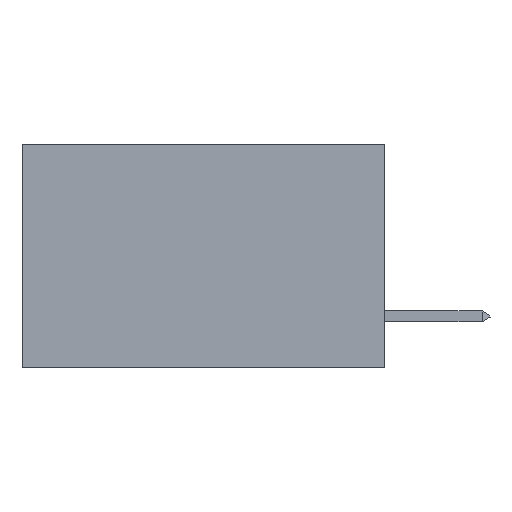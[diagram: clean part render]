
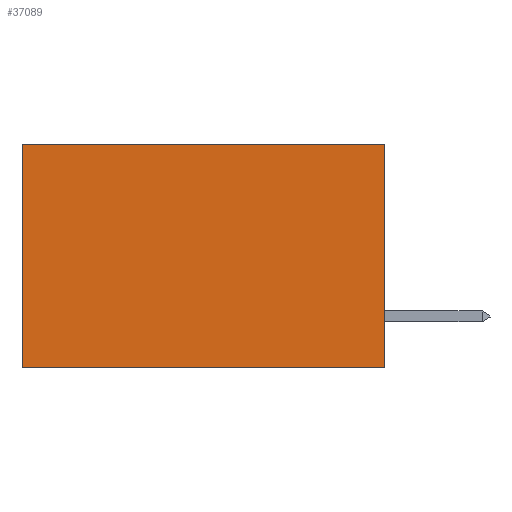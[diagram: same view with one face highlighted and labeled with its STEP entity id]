
A CAD part, left-side view. The second image highlights one B-rep face of the part: STEP entity #37089.
In plain terms, the highlighted planar face has unit normal (-1, 0, 0).
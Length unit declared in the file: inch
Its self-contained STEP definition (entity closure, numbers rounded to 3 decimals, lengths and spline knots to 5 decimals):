
#226 = VERTEX_POINT ( 'NONE', #22843 ) ;
#291 = EDGE_CURVE ( 'NONE', #226, #2371, #13985, .T. ) ;
#1689 = EDGE_CURVE ( 'NONE', #10957, #2266, #26819, .T. ) ;
#2266 = VERTEX_POINT ( 'NONE', #9314 ) ;
#2371 = VERTEX_POINT ( 'NONE', #36547 ) ;
#2788 = ORIENTED_EDGE ( 'NONE', *, *, #1689, .F. ) ;
#2862 = DIRECTION ( 'NONE',  ( 0., 1., 0. ) ) ;
#5697 = LINE ( 'NONE', #27568, #25083 ) ;
#6122 = VECTOR ( 'NONE', #29464, 39.37008 ) ;
#6258 = EDGE_CURVE ( 'NONE', #226, #10957, #12650, .T. ) ;
#7925 = VECTOR ( 'NONE', #2862, 39.37008 ) ;
#8088 = CARTESIAN_POINT ( 'NONE',  ( 0.2875, 0., 0. ) ) ;
#9281 = CARTESIAN_POINT ( 'NONE',  ( 0.2875, 0., 0. ) ) ;
#9314 = CARTESIAN_POINT ( 'NONE',  ( 0.2875, 0.6, -0.37 ) ) ;
#9414 = DIRECTION ( 'NONE',  ( 1., 0., 0. ) ) ;
#9442 = VECTOR ( 'NONE', #23203, 39.37008 ) ;
#10364 = EDGE_CURVE ( 'NONE', #2371, #2266, #5697, .T. ) ;
#10585 = AXIS2_PLACEMENT_3D ( 'NONE', #9281, #9414, #29899 ) ;
#10957 = VERTEX_POINT ( 'NONE', #12970 ) ;
#12650 = LINE ( 'NONE', #8088, #9442 ) ;
#12970 = CARTESIAN_POINT ( 'NONE',  ( 0.2875, 0., -0.37 ) ) ;
#13985 = LINE ( 'NONE', #15179, #6122 ) ;
#15107 = PLANE ( 'NONE',  #10585 ) ;
#15179 = CARTESIAN_POINT ( 'NONE',  ( 0.2875, 0., 0. ) ) ;
#18795 = ORIENTED_EDGE ( 'NONE', *, *, #10364, .T. ) ;
#22798 = DIRECTION ( 'NONE',  ( 0., 0., -1. ) ) ;
#22843 = CARTESIAN_POINT ( 'NONE',  ( 0.2875, 0., 0. ) ) ;
#23203 = DIRECTION ( 'NONE',  ( 0., 0., -1. ) ) ;
#25083 = VECTOR ( 'NONE', #22798, 39.37008 ) ;
#26819 = LINE ( 'NONE', #27489, #7925 ) ;
#27489 = CARTESIAN_POINT ( 'NONE',  ( 0.2875, 0., -0.37 ) ) ;
#27568 = CARTESIAN_POINT ( 'NONE',  ( 0.2875, 0.6, 0. ) ) ;
#29464 = DIRECTION ( 'NONE',  ( 0., 1., 0. ) ) ;
#29899 = DIRECTION ( 'NONE',  ( 0., 0., -1. ) ) ;
#34164 = EDGE_LOOP ( 'NONE', ( #18795, #2788, #36025, #37506 ) ) ;
#34570 = FACE_OUTER_BOUND ( 'NONE', #34164, .T. ) ;
#36025 = ORIENTED_EDGE ( 'NONE', *, *, #6258, .F. ) ;
#36547 = CARTESIAN_POINT ( 'NONE',  ( 0.2875, 0.6, 0. ) ) ;
#37089 = ADVANCED_FACE ( 'NONE', ( #34570 ), #15107, .F. ) ;
#37506 = ORIENTED_EDGE ( 'NONE', *, *, #291, .T. ) ;
